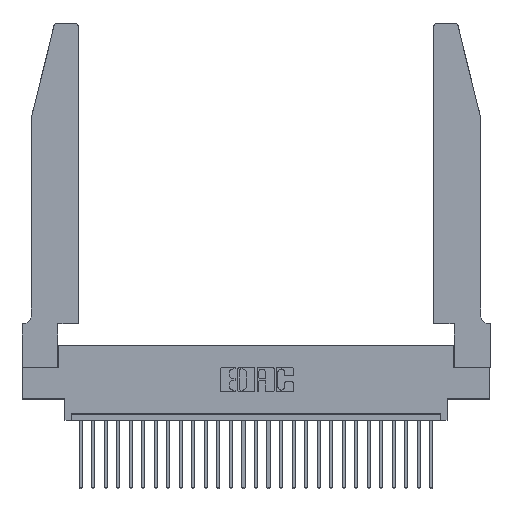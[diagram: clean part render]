
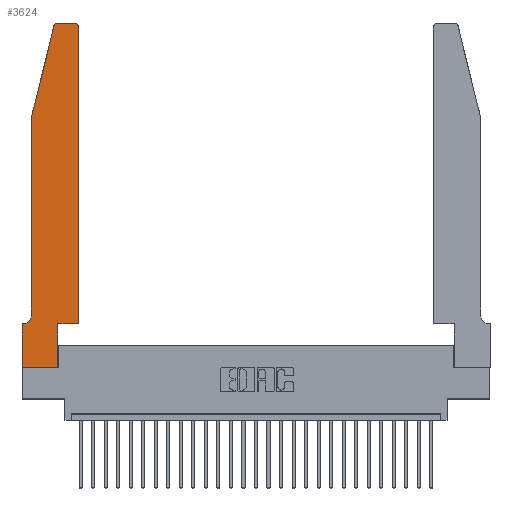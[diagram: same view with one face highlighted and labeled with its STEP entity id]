
A CAD part, top view. The second image highlights one B-rep face of the part: STEP entity #3624.
In plain terms, the highlighted planar face has unit normal (0, 0, 1).
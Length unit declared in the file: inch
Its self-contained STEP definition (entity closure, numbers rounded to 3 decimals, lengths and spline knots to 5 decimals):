
#44 = CARTESIAN_POINT ( 'NONE',  ( 0., 0.35, 0.37 ) ) ;
#258 = CIRCLE ( 'NONE', #26884, 0.03 ) ;
#481 = ORIENTED_EDGE ( 'NONE', *, *, #21953, .T. ) ;
#847 = EDGE_CURVE ( 'NONE', #17770, #1505, #15962, .T. ) ;
#1222 = VERTEX_POINT ( 'NONE', #1801 ) ;
#1325 = LINE ( 'NONE', #16424, #8290 ) ;
#1505 = VERTEX_POINT ( 'NONE', #27680 ) ;
#1801 = CARTESIAN_POINT ( 'NONE',  ( 0.4205, 2.75, 0.37 ) ) ;
#1803 = VECTOR ( 'NONE', #8695, 39.37008 ) ;
#1980 = EDGE_LOOP ( 'NONE', ( #27931, #22796, #21517, #481, #10991, #26754, #9400, #12083, #12599, #20468, #11512, #16093 ) ) ;
#2658 = DIRECTION ( 'NONE',  ( 0., -1., 0. ) ) ;
#3055 = AXIS2_PLACEMENT_3D ( 'NONE', #44, #13645, #22052 ) ;
#3097 = EDGE_CURVE ( 'NONE', #5790, #27250, #6229, .T. ) ;
#3624 = ADVANCED_FACE ( 'NONE', ( #28191 ), #20000, .T. ) ;
#3768 = EDGE_CURVE ( 'NONE', #18658, #5790, #4102, .T. ) ;
#3874 = VECTOR ( 'NONE', #8075, 39.37008 ) ;
#3975 = CARTESIAN_POINT ( 'NONE',  ( 0.2865, 0.35, 0.37 ) ) ;
#4061 = DIRECTION ( 'NONE',  ( 1., 0., 0. ) ) ;
#4102 = CIRCLE ( 'NONE', #10097, 0.03 ) ;
#4234 = CARTESIAN_POINT ( 'NONE',  ( 0., 0., 0.37 ) ) ;
#4284 = VERTEX_POINT ( 'NONE', #3975 ) ;
#4604 = CARTESIAN_POINT ( 'NONE',  ( 0.2865, 0., 0.37 ) ) ;
#4742 = CIRCLE ( 'NONE', #26829, 0.07 ) ;
#4830 = CARTESIAN_POINT ( 'NONE',  ( 0.4505, 0.35, 0.37 ) ) ;
#5210 = CARTESIAN_POINT ( 'NONE',  ( 0., 0., 0.37 ) ) ;
#5790 = VERTEX_POINT ( 'NONE', #16431 ) ;
#5864 = DIRECTION ( 'NONE',  ( -1., 0., 0. ) ) ;
#6127 = DIRECTION ( 'NONE',  ( 0., 0., 1. ) ) ;
#6205 = CARTESIAN_POINT ( 'NONE',  ( 0.4205, 2.72, 0.37 ) ) ;
#6229 = LINE ( 'NONE', #8636, #8984 ) ;
#6990 = LINE ( 'NONE', #19559, #1803 ) ;
#7102 = LINE ( 'NONE', #19335, #10578 ) ;
#7926 = CARTESIAN_POINT ( 'NONE',  ( 0.0755, 2., 0.37 ) ) ;
#8075 = DIRECTION ( 'NONE',  ( -1., 0., 0. ) ) ;
#8290 = VECTOR ( 'NONE', #27468, 39.37008 ) ;
#8447 = DIRECTION ( 'NONE',  ( 1., 0., 0. ) ) ;
#8636 = CARTESIAN_POINT ( 'NONE',  ( 0.0755, 2., 0.37 ) ) ;
#8695 = DIRECTION ( 'NONE',  ( 0., 1., 0. ) ) ;
#8984 = VECTOR ( 'NONE', #9470, 39.37008 ) ;
#9076 = EDGE_CURVE ( 'NONE', #15777, #25297, #13194, .T. ) ;
#9331 = CARTESIAN_POINT ( 'NONE',  ( 0.0755, 2., 0.37 ) ) ;
#9400 = ORIENTED_EDGE ( 'NONE', *, *, #13487, .T. ) ;
#9470 = DIRECTION ( 'NONE',  ( -0.239, -0.971, 0. ) ) ;
#9528 = VECTOR ( 'NONE', #2658, 39.37008 ) ;
#9715 = CARTESIAN_POINT ( 'NONE',  ( 0.4505, 2.72, 0.37 ) ) ;
#10097 = AXIS2_PLACEMENT_3D ( 'NONE', #17157, #6127, #8447 ) ;
#10578 = VECTOR ( 'NONE', #5864, 39.37008 ) ;
#10622 = VERTEX_POINT ( 'NONE', #4234 ) ;
#10991 = ORIENTED_EDGE ( 'NONE', *, *, #12895, .T. ) ;
#11171 = VERTEX_POINT ( 'NONE', #28119 ) ;
#11505 = LINE ( 'NONE', #22460, #22503 ) ;
#11512 = ORIENTED_EDGE ( 'NONE', *, *, #9076, .T. ) ;
#12083 = ORIENTED_EDGE ( 'NONE', *, *, #17506, .T. ) ;
#12144 = EDGE_CURVE ( 'NONE', #4284, #15777, #1325, .T. ) ;
#12599 = ORIENTED_EDGE ( 'NONE', *, *, #24314, .T. ) ;
#12895 = EDGE_CURVE ( 'NONE', #11171, #17770, #4742, .T. ) ;
#13194 = LINE ( 'NONE', #4830, #27972 ) ;
#13487 = EDGE_CURVE ( 'NONE', #1505, #10622, #16750, .T. ) ;
#13645 = DIRECTION ( 'NONE',  ( 0., 0., 1. ) ) ;
#14767 = CARTESIAN_POINT ( 'NONE',  ( 0.0755, 0.35, 0.37 ) ) ;
#15031 = VECTOR ( 'NONE', #24590, 39.37008 ) ;
#15712 = EDGE_CURVE ( 'NONE', #1222, #18658, #7102, .T. ) ;
#15777 = VERTEX_POINT ( 'NONE', #19618 ) ;
#15962 = LINE ( 'NONE', #14767, #3874 ) ;
#16093 = ORIENTED_EDGE ( 'NONE', *, *, #26674, .T. ) ;
#16352 = CARTESIAN_POINT ( 'NONE',  ( 0.284, 2.75, 0.37 ) ) ;
#16424 = CARTESIAN_POINT ( 'NONE',  ( 0.4505, 0.35, 0.37 ) ) ;
#16431 = CARTESIAN_POINT ( 'NONE',  ( 0.25487, 2.72718, 0.37 ) ) ;
#16750 = LINE ( 'NONE', #5210, #15031 ) ;
#17157 = CARTESIAN_POINT ( 'NONE',  ( 0.284, 2.72, 0.37 ) ) ;
#17506 = EDGE_CURVE ( 'NONE', #10622, #18798, #11505, .T. ) ;
#17770 = VERTEX_POINT ( 'NONE', #19067 ) ;
#18658 = VERTEX_POINT ( 'NONE', #16352 ) ;
#18798 = VERTEX_POINT ( 'NONE', #4604 ) ;
#19067 = CARTESIAN_POINT ( 'NONE',  ( 0.0055, 0.35, 0.37 ) ) ;
#19335 = CARTESIAN_POINT ( 'NONE',  ( 0.2605, 2.75, 0.37 ) ) ;
#19559 = CARTESIAN_POINT ( 'NONE',  ( 0.2865, 0.35, 0.37 ) ) ;
#19618 = CARTESIAN_POINT ( 'NONE',  ( 0.4505, 0.35, 0.37 ) ) ;
#20000 = PLANE ( 'NONE',  #3055 ) ;
#20266 = DIRECTION ( 'NONE',  ( 0., 1., 0. ) ) ;
#20468 = ORIENTED_EDGE ( 'NONE', *, *, #12144, .T. ) ;
#21517 = ORIENTED_EDGE ( 'NONE', *, *, #3097, .T. ) ;
#21953 = EDGE_CURVE ( 'NONE', #27250, #11171, #26342, .T. ) ;
#22052 = DIRECTION ( 'NONE',  ( 1., 0., 0. ) ) ;
#22460 = CARTESIAN_POINT ( 'NONE',  ( 0., 0., 0.37 ) ) ;
#22503 = VECTOR ( 'NONE', #25735, 39.37008 ) ;
#22796 = ORIENTED_EDGE ( 'NONE', *, *, #3768, .T. ) ;
#24314 = EDGE_CURVE ( 'NONE', #18798, #4284, #6990, .T. ) ;
#24590 = DIRECTION ( 'NONE',  ( 0., -1., 0. ) ) ;
#25297 = VERTEX_POINT ( 'NONE', #9715 ) ;
#25701 = DIRECTION ( 'NONE',  ( 0., 0., 1. ) ) ;
#25735 = DIRECTION ( 'NONE',  ( 1., 0., 0. ) ) ;
#25757 = CARTESIAN_POINT ( 'NONE',  ( 0.0055, 0.42, 0.37 ) ) ;
#26342 = LINE ( 'NONE', #9331, #9528 ) ;
#26674 = EDGE_CURVE ( 'NONE', #25297, #1222, #258, .T. ) ;
#26754 = ORIENTED_EDGE ( 'NONE', *, *, #847, .T. ) ;
#26829 = AXIS2_PLACEMENT_3D ( 'NONE', #25757, #28352, #28153 ) ;
#26884 = AXIS2_PLACEMENT_3D ( 'NONE', #6205, #25701, #4061 ) ;
#27250 = VERTEX_POINT ( 'NONE', #7926 ) ;
#27468 = DIRECTION ( 'NONE',  ( 1., 0., 0. ) ) ;
#27680 = CARTESIAN_POINT ( 'NONE',  ( 0., 0.35, 0.37 ) ) ;
#27931 = ORIENTED_EDGE ( 'NONE', *, *, #15712, .T. ) ;
#27972 = VECTOR ( 'NONE', #20266, 39.37008 ) ;
#28119 = CARTESIAN_POINT ( 'NONE',  ( 0.0755, 0.42, 0.37 ) ) ;
#28153 = DIRECTION ( 'NONE',  ( -1., 0., 0. ) ) ;
#28191 = FACE_OUTER_BOUND ( 'NONE', #1980, .T. ) ;
#28352 = DIRECTION ( 'NONE',  ( 0., 0., -1. ) ) ;
